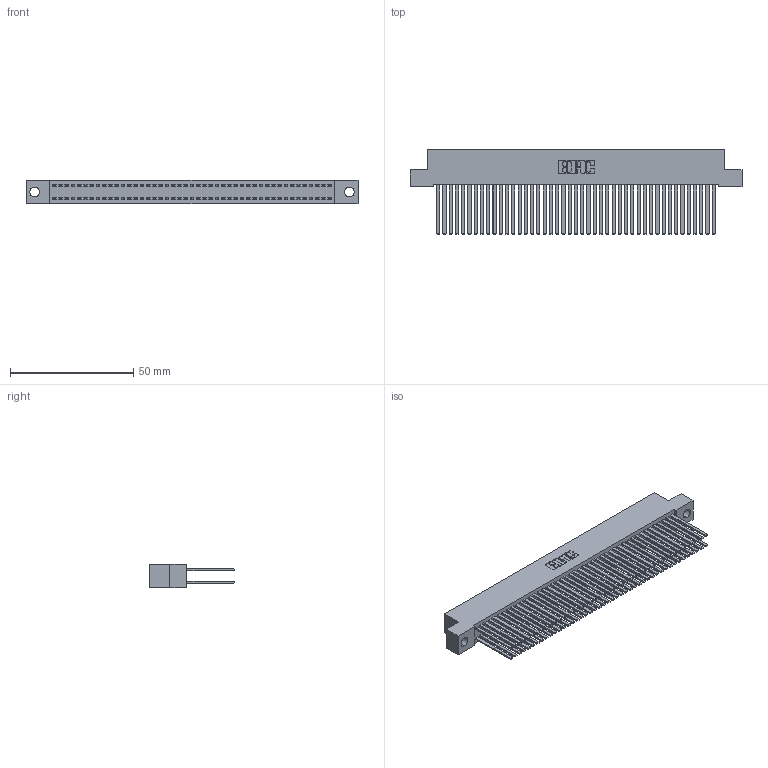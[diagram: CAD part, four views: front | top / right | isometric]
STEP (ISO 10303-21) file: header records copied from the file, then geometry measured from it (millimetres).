
FILE_DESCRIPTION (( 'STEP AP203' ), '1' );
FILE_NAME ('392-090-544-204.STEP', '2019-10-09T18:31:13', ( '' ), ( '' ), 'SwSTEP 2.0', 'SolidWorks 2016', '' );
FILE_SCHEMA (( 'CONFIG_CONTROL_DESIGN' ));
Length unit declared in the file: inch
Products named in the file (3): 345-292-001_345-293-144; 392-090-544-204; 342 Part_.156 TH
Assembly tree (91 placements, depth 2):
  392-090-544-204
    342 Part_.156 TH
    345-292-001_345-293-144  x90
Bounding box: 134.62 x 34.3 x 9.4 mm (x, y, z)
Volume: 13284.4 mm3; surface area: 25015.7 mm2
Topology: 91 solids, 91 shells, 4250 faces, 12629 edges, 8298 vertices
Faces by surface type: plane 2946, cylinder 1304
Entity records: 28249 total; most frequent: CARTESIAN_POINT 4674, ORIENTED_EDGE 4610, DIRECTION 3985, EDGE_CURVE 2305, VECTOR 2181, LINE 2181, VERTEX_POINT 1534, AXIS2_PLACEMENT_3D 902
